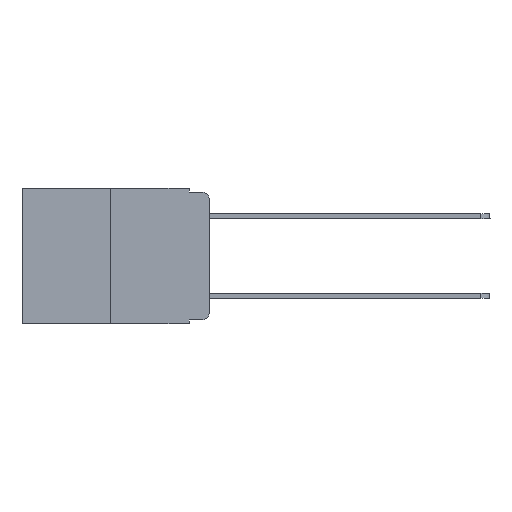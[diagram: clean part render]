
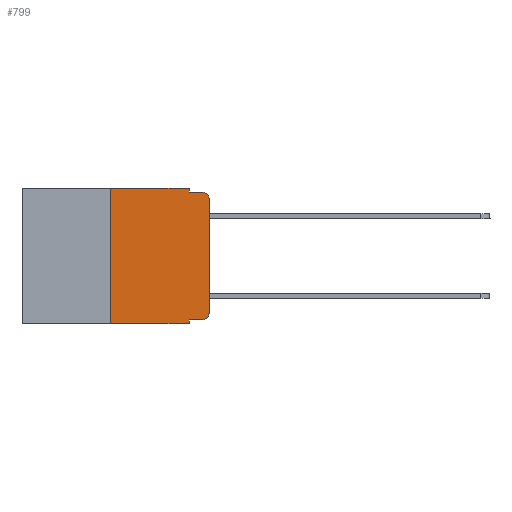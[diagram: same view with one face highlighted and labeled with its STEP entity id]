
A CAD part, left-side view. The second image highlights one B-rep face of the part: STEP entity #799.
In plain terms, the highlighted planar face has unit normal (-1, 0, 0).
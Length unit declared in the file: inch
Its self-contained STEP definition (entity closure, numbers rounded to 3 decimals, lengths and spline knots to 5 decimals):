
#221 = ORIENTED_EDGE ( 'NONE', *, *, #14985, .F. ) ;
#302 = VECTOR ( 'NONE', #20753, 39.37008 ) ;
#799 = ADVANCED_FACE ( 'NONE', ( #17674 ), #4261, .F. ) ;
#1507 = CARTESIAN_POINT ( 'NONE',  ( 0., 0.02, -0.03 ) ) ;
#1593 = DIRECTION ( 'NONE',  ( 0., -1., 0. ) ) ;
#1632 = EDGE_CURVE ( 'NONE', #14454, #15272, #18524, .T. ) ;
#2299 = ORIENTED_EDGE ( 'NONE', *, *, #4147, .F. ) ;
#2589 = EDGE_CURVE ( 'NONE', #9733, #8062, #15279, .T. ) ;
#2613 = DIRECTION ( 'NONE',  ( -1., 0., 0. ) ) ;
#2646 = CARTESIAN_POINT ( 'NONE',  ( 0., 0.473, -0.343 ) ) ;
#2719 = CARTESIAN_POINT ( 'NONE',  ( 0., 0.473, 0. ) ) ;
#2875 = AXIS2_PLACEMENT_3D ( 'NONE', #1507, #23687, #3530 ) ;
#3087 = CARTESIAN_POINT ( 'NONE',  ( 0., 0., -0.313 ) ) ;
#3530 = DIRECTION ( 'NONE',  ( 0., 0., -1. ) ) ;
#3596 = AXIS2_PLACEMENT_3D ( 'NONE', #6247, #2613, #8111 ) ;
#3865 = CARTESIAN_POINT ( 'NONE',  ( 0., 0.02, -0.01 ) ) ;
#4147 = EDGE_CURVE ( 'NONE', #4733, #14454, #21617, .T. ) ;
#4234 = ORIENTED_EDGE ( 'NONE', *, *, #23131, .F. ) ;
#4261 = PLANE ( 'NONE',  #5210 ) ;
#4596 = LINE ( 'NONE', #12896, #11268 ) ;
#4733 = VERTEX_POINT ( 'NONE', #12682 ) ;
#5071 = EDGE_CURVE ( 'NONE', #16793, #19849, #10290, .T. ) ;
#5210 = AXIS2_PLACEMENT_3D ( 'NONE', #2719, #14198, #13872 ) ;
#5400 = VECTOR ( 'NONE', #15578, 39.37008 ) ;
#5639 = CARTESIAN_POINT ( 'NONE',  ( 0., 0.051, -0.01 ) ) ;
#5949 = LINE ( 'NONE', #2646, #5400 ) ;
#5984 = CARTESIAN_POINT ( 'NONE',  ( 0., 0.051, 0. ) ) ;
#6227 = EDGE_CURVE ( 'NONE', #4733, #13680, #5949, .T. ) ;
#6238 = ORIENTED_EDGE ( 'NONE', *, *, #12673, .T. ) ;
#6247 = CARTESIAN_POINT ( 'NONE',  ( 0., 0.02, -0.313 ) ) ;
#6287 = VECTOR ( 'NONE', #18604, 39.37008 ) ;
#6369 = CARTESIAN_POINT ( 'NONE',  ( 0., 0.25, 0. ) ) ;
#6843 = VECTOR ( 'NONE', #9706, 39.37008 ) ;
#7009 = CARTESIAN_POINT ( 'NONE',  ( 0., 0.051, -0.333 ) ) ;
#8062 = VERTEX_POINT ( 'NONE', #3865 ) ;
#8111 = DIRECTION ( 'NONE',  ( 0., 0., -1. ) ) ;
#8692 = CARTESIAN_POINT ( 'NONE',  ( 0., 0.051, -0.01 ) ) ;
#8999 = DIRECTION ( 'NONE',  ( 0., 0., -1. ) ) ;
#9209 = DIRECTION ( 'NONE',  ( 0., -1., 0. ) ) ;
#9706 = DIRECTION ( 'NONE',  ( 0., 0., 1. ) ) ;
#9733 = VERTEX_POINT ( 'NONE', #18479 ) ;
#10290 = CIRCLE ( 'NONE', #3596, 0.02 ) ;
#10342 = EDGE_CURVE ( 'NONE', #16624, #8062, #13250, .T. ) ;
#10357 = EDGE_LOOP ( 'NONE', ( #6238, #18661, #13080, #221, #19161, #2299, #13323, #4234, #13031, #15876 ) ) ;
#11268 = VECTOR ( 'NONE', #8999, 39.37008 ) ;
#12380 = CARTESIAN_POINT ( 'NONE',  ( 0., 0., 0. ) ) ;
#12673 = EDGE_CURVE ( 'NONE', #19849, #9733, #19212, .T. ) ;
#12682 = CARTESIAN_POINT ( 'NONE',  ( 0., 0.25, -0.343 ) ) ;
#12767 = EDGE_CURVE ( 'NONE', #19773, #16793, #21206, .T. ) ;
#12896 = CARTESIAN_POINT ( 'NONE',  ( 0., 0.051, 0. ) ) ;
#13031 = ORIENTED_EDGE ( 'NONE', *, *, #12767, .T. ) ;
#13080 = ORIENTED_EDGE ( 'NONE', *, *, #10342, .F. ) ;
#13250 = LINE ( 'NONE', #5639, #22522 ) ;
#13323 = ORIENTED_EDGE ( 'NONE', *, *, #6227, .T. ) ;
#13521 = CARTESIAN_POINT ( 'NONE',  ( 0., 0.051, -0.333 ) ) ;
#13680 = VERTEX_POINT ( 'NONE', #15134 ) ;
#13872 = DIRECTION ( 'NONE',  ( 0., 0., -1. ) ) ;
#14113 = LINE ( 'NONE', #14662, #6287 ) ;
#14198 = DIRECTION ( 'NONE',  ( 1., 0., 0. ) ) ;
#14454 = VERTEX_POINT ( 'NONE', #6369 ) ;
#14662 = CARTESIAN_POINT ( 'NONE',  ( 0., 0.051, 0. ) ) ;
#14985 = EDGE_CURVE ( 'NONE', #15272, #16624, #4596, .T. ) ;
#15134 = CARTESIAN_POINT ( 'NONE',  ( 0., 0.051, -0.343 ) ) ;
#15192 = CARTESIAN_POINT ( 'NONE',  ( 0., 0.25, 0. ) ) ;
#15272 = VERTEX_POINT ( 'NONE', #5984 ) ;
#15279 = CIRCLE ( 'NONE', #2875, 0.02 ) ;
#15578 = DIRECTION ( 'NONE',  ( 0., -1., 0. ) ) ;
#15876 = ORIENTED_EDGE ( 'NONE', *, *, #5071, .T. ) ;
#16260 = CARTESIAN_POINT ( 'NONE',  ( 0., 0.02, -0.333 ) ) ;
#16624 = VERTEX_POINT ( 'NONE', #8692 ) ;
#16793 = VERTEX_POINT ( 'NONE', #16260 ) ;
#17674 = FACE_OUTER_BOUND ( 'NONE', #10357, .T. ) ;
#17989 = DIRECTION ( 'NONE',  ( 0., 0., 1. ) ) ;
#18289 = VECTOR ( 'NONE', #1593, 39.37008 ) ;
#18479 = CARTESIAN_POINT ( 'NONE',  ( 0., 0., -0.03 ) ) ;
#18524 = LINE ( 'NONE', #20910, #302 ) ;
#18604 = DIRECTION ( 'NONE',  ( 0., 0., -1. ) ) ;
#18661 = ORIENTED_EDGE ( 'NONE', *, *, #2589, .T. ) ;
#19161 = ORIENTED_EDGE ( 'NONE', *, *, #1632, .F. ) ;
#19212 = LINE ( 'NONE', #12380, #21834 ) ;
#19773 = VERTEX_POINT ( 'NONE', #13521 ) ;
#19849 = VERTEX_POINT ( 'NONE', #3087 ) ;
#20753 = DIRECTION ( 'NONE',  ( 0., -1., 0. ) ) ;
#20910 = CARTESIAN_POINT ( 'NONE',  ( 0., 0.473, 0. ) ) ;
#21206 = LINE ( 'NONE', #7009, #18289 ) ;
#21617 = LINE ( 'NONE', #15192, #6843 ) ;
#21834 = VECTOR ( 'NONE', #17989, 39.37008 ) ;
#22522 = VECTOR ( 'NONE', #9209, 39.37008 ) ;
#23131 = EDGE_CURVE ( 'NONE', #19773, #13680, #14113, .T. ) ;
#23687 = DIRECTION ( 'NONE',  ( -1., 0., 0. ) ) ;
